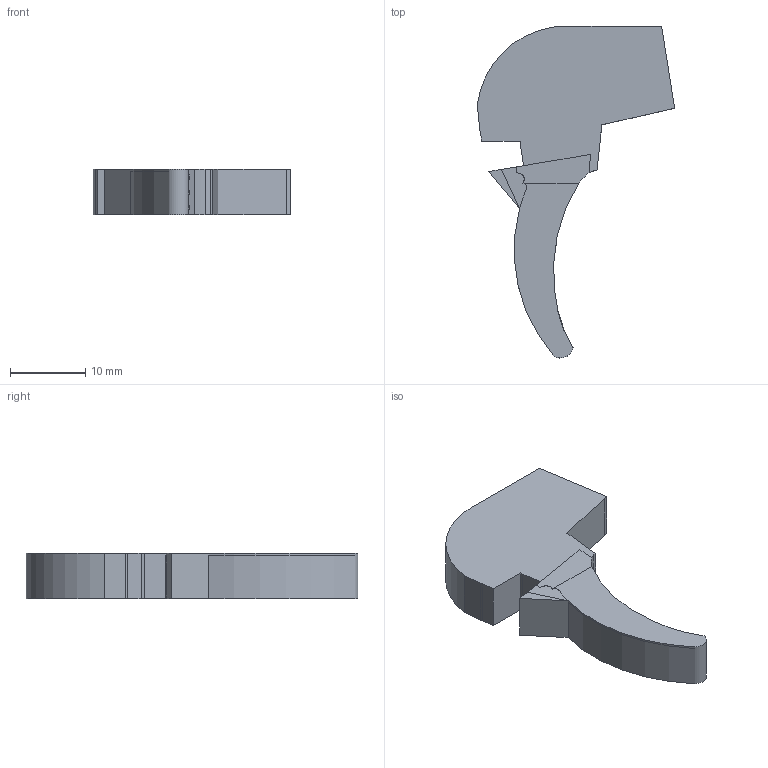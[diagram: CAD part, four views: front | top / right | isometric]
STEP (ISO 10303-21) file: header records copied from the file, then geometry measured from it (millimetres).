
FILE_DESCRIPTION(/* description */ (''),/* implementation_level */ '2;1');
FILE_NAME(/* name */ '',/* time_stamp */ '',/* author */ (''),/* organization */ (''),/* preprocessor_version */ 'ST-DEVELOPER v18.1',/* originating_system */ 'Autodesk Translation Framework v9.7.1.1290',/* authorisation */ '');
FILE_SCHEMA (('AUTOMOTIVE_DESIGN { 1 0 10303 214 3 1 1 }'));
Length unit declared in the file: millimetre
Products named in the file (1): Trigger (Printable) (1)
Bounding box: 26.27 x 44.17 x 6 mm (x, y, z)
Volume: 3078.2 mm3; surface area: 1818.2 mm2
Topology: 1 solids, 1 shells, 48 faces, 134 edges, 90 vertices
Faces by surface type: plane 33, cylinder 10, bspline 5
Entity records: 1804 total; most frequent: CARTESIAN_POINT 612, ORIENTED_EDGE 268, DIRECTION 198, EDGE_CURVE 134, VERTEX_POINT 90, LINE 78, VECTOR 78, AXIS2_PLACEMENT_3D 60
